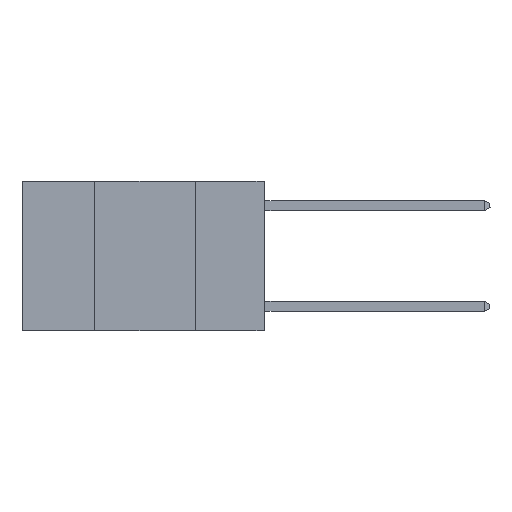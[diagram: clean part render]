
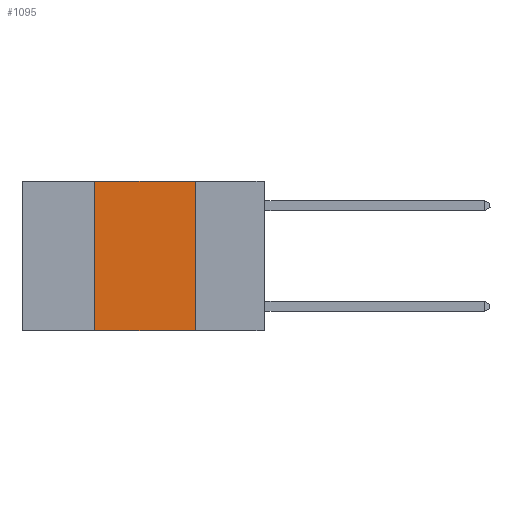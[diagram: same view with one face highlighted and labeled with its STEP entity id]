
A CAD part, left-side view. The second image highlights one B-rep face of the part: STEP entity #1095.
In plain terms, the highlighted planar face has unit normal (-1, 0, 0).
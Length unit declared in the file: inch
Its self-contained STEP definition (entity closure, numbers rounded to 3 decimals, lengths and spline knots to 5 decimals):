
#119 = FACE_OUTER_BOUND ( 'NONE', #8440, .T. ) ;
#485 = CARTESIAN_POINT ( 'NONE',  ( 0., 0.17, -0.37 ) ) ;
#802 = LINE ( 'NONE', #10563, #5083 ) ;
#1010 = CARTESIAN_POINT ( 'NONE',  ( 0., 0.6, 0. ) ) ;
#1095 = ADVANCED_FACE ( 'NONE', ( #119 ), #3034, .F. ) ;
#1393 = VECTOR ( 'NONE', #7033, 39.37008 ) ;
#1980 = DIRECTION ( 'NONE',  ( 0., 0., -1. ) ) ;
#2026 = VERTEX_POINT ( 'NONE', #9154 ) ;
#2038 = DIRECTION ( 'NONE',  ( 1., 0., 0. ) ) ;
#2262 = CARTESIAN_POINT ( 'NONE',  ( 0., 0.42, 0. ) ) ;
#3034 = PLANE ( 'NONE',  #4225 ) ;
#3261 = CARTESIAN_POINT ( 'NONE',  ( 0., 0.6, -0.37 ) ) ;
#3420 = VERTEX_POINT ( 'NONE', #8287 ) ;
#3723 = EDGE_CURVE ( 'NONE', #2026, #4826, #7905, .T. ) ;
#4225 = AXIS2_PLACEMENT_3D ( 'NONE', #1010, #2038, #1980 ) ;
#4826 = VERTEX_POINT ( 'NONE', #485 ) ;
#4972 = LINE ( 'NONE', #3261, #10146 ) ;
#5018 = DIRECTION ( 'NONE',  ( 0., 0., -1. ) ) ;
#5061 = EDGE_CURVE ( 'NONE', #3420, #6985, #7906, .T. ) ;
#5071 = CARTESIAN_POINT ( 'NONE',  ( 0., 0.42, 0. ) ) ;
#5083 = VECTOR ( 'NONE', #5722, 39.37008 ) ;
#5722 = DIRECTION ( 'NONE',  ( 0., -1., 0. ) ) ;
#6706 = EDGE_CURVE ( 'NONE', #6985, #2026, #802, .T. ) ;
#6985 = VERTEX_POINT ( 'NONE', #5071 ) ;
#7033 = DIRECTION ( 'NONE',  ( 0., 0., 1. ) ) ;
#7442 = ORIENTED_EDGE ( 'NONE', *, *, #6706, .F. ) ;
#7548 = ORIENTED_EDGE ( 'NONE', *, *, #5061, .F. ) ;
#7676 = EDGE_CURVE ( 'NONE', #3420, #4826, #4972, .T. ) ;
#7905 = LINE ( 'NONE', #10938, #11599 ) ;
#7906 = LINE ( 'NONE', #2262, #1393 ) ;
#8287 = CARTESIAN_POINT ( 'NONE',  ( 0., 0.42, -0.37 ) ) ;
#8292 = ORIENTED_EDGE ( 'NONE', *, *, #3723, .F. ) ;
#8440 = EDGE_LOOP ( 'NONE', ( #8292, #7442, #7548, #11529 ) ) ;
#8804 = DIRECTION ( 'NONE',  ( 0., -1., 0. ) ) ;
#9154 = CARTESIAN_POINT ( 'NONE',  ( 0., 0.17, 0. ) ) ;
#10146 = VECTOR ( 'NONE', #8804, 39.37008 ) ;
#10563 = CARTESIAN_POINT ( 'NONE',  ( 0., 0.6, 0. ) ) ;
#10938 = CARTESIAN_POINT ( 'NONE',  ( 0., 0.17, 0. ) ) ;
#11529 = ORIENTED_EDGE ( 'NONE', *, *, #7676, .T. ) ;
#11599 = VECTOR ( 'NONE', #5018, 39.37008 ) ;
